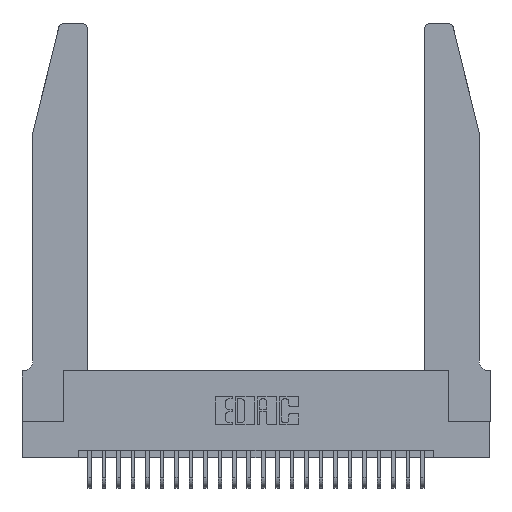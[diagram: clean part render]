
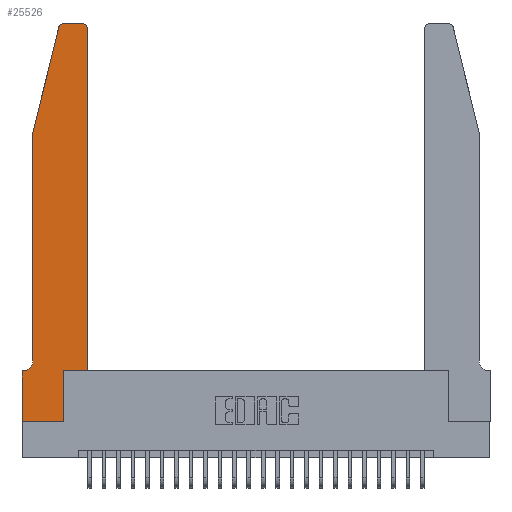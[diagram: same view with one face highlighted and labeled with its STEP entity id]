
A CAD part, top view. The second image highlights one B-rep face of the part: STEP entity #25526.
In plain terms, the highlighted planar face has unit normal (0, 0, 1).
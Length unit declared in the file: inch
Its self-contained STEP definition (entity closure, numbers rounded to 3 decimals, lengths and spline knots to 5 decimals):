
#238 = CARTESIAN_POINT ( 'NONE',  ( 0.2865, 0.35, 0.37 ) ) ;
#315 = ORIENTED_EDGE ( 'NONE', *, *, #3221, .T. ) ;
#940 = DIRECTION ( 'NONE',  ( -0.239, -0.971, 0. ) ) ;
#980 = LINE ( 'NONE', #2149, #10049 ) ;
#1120 = ORIENTED_EDGE ( 'NONE', *, *, #13554, .T. ) ;
#1288 = ORIENTED_EDGE ( 'NONE', *, *, #10608, .T. ) ;
#1357 = VECTOR ( 'NONE', #27537, 39.37008 ) ;
#1616 = CIRCLE ( 'NONE', #3558, 0.03 ) ;
#2002 = ORIENTED_EDGE ( 'NONE', *, *, #13219, .T. ) ;
#2116 = DIRECTION ( 'NONE',  ( 0., -1., 0. ) ) ;
#2149 = CARTESIAN_POINT ( 'NONE',  ( 0.4505, 0.35, 0.37 ) ) ;
#2176 = CARTESIAN_POINT ( 'NONE',  ( 0., 0., 0.37 ) ) ;
#2325 = ORIENTED_EDGE ( 'NONE', *, *, #15446, .T. ) ;
#2406 = EDGE_CURVE ( 'NONE', #17965, #20600, #19378, .T. ) ;
#3221 = EDGE_CURVE ( 'NONE', #5025, #9266, #23312, .T. ) ;
#3550 = VERTEX_POINT ( 'NONE', #16553 ) ;
#3558 = AXIS2_PLACEMENT_3D ( 'NONE', #22043, #26287, #18060 ) ;
#3704 = DIRECTION ( 'NONE',  ( 0., 1., 0. ) ) ;
#4265 = EDGE_CURVE ( 'NONE', #22659, #5025, #15435, .T. ) ;
#4326 = CARTESIAN_POINT ( 'NONE',  ( 0., 0.35, 0.37 ) ) ;
#4814 = LINE ( 'NONE', #26603, #12857 ) ;
#4916 = CARTESIAN_POINT ( 'NONE',  ( 0.4505, 2.72, 0.37 ) ) ;
#4951 = VECTOR ( 'NONE', #3704, 39.37008 ) ;
#5025 = VERTEX_POINT ( 'NONE', #4326 ) ;
#5182 = CARTESIAN_POINT ( 'NONE',  ( 0.0755, 2., 0.37 ) ) ;
#5240 = ORIENTED_EDGE ( 'NONE', *, *, #4265, .T. ) ;
#5340 = LINE ( 'NONE', #8900, #21389 ) ;
#6276 = DIRECTION ( 'NONE',  ( 0., 0., -1. ) ) ;
#8900 = CARTESIAN_POINT ( 'NONE',  ( 0.4505, 0.35, 0.37 ) ) ;
#8917 = CIRCLE ( 'NONE', #25236, 0.03 ) ;
#9266 = VERTEX_POINT ( 'NONE', #20901 ) ;
#9493 = CARTESIAN_POINT ( 'NONE',  ( 0.0055, 0.35, 0.37 ) ) ;
#9686 = ORIENTED_EDGE ( 'NONE', *, *, #2406, .T. ) ;
#10049 = VECTOR ( 'NONE', #25887, 39.37008 ) ;
#10050 = CARTESIAN_POINT ( 'NONE',  ( 0.4505, 0.35, 0.37 ) ) ;
#10266 = CARTESIAN_POINT ( 'NONE',  ( 0., 0., 0.37 ) ) ;
#10285 = EDGE_CURVE ( 'NONE', #14679, #10749, #21225, .T. ) ;
#10608 = EDGE_CURVE ( 'NONE', #19831, #22659, #23866, .T. ) ;
#10749 = VERTEX_POINT ( 'NONE', #20381 ) ;
#10886 = EDGE_CURVE ( 'NONE', #3550, #19831, #4814, .T. ) ;
#11012 = VERTEX_POINT ( 'NONE', #11297 ) ;
#11286 = EDGE_LOOP ( 'NONE', ( #25298, #2325, #15793, #12590, #1288, #5240, #315, #16983, #9686, #2002, #1120, #18285 ) ) ;
#11297 = CARTESIAN_POINT ( 'NONE',  ( 0.25487, 2.72718, 0.37 ) ) ;
#11981 = VECTOR ( 'NONE', #2116, 39.37008 ) ;
#12291 = EDGE_CURVE ( 'NONE', #9266, #17965, #23465, .T. ) ;
#12590 = ORIENTED_EDGE ( 'NONE', *, *, #10886, .T. ) ;
#12857 = VECTOR ( 'NONE', #13670, 39.37008 ) ;
#12926 = DIRECTION ( 'NONE',  ( 0., 0., 1. ) ) ;
#13219 = EDGE_CURVE ( 'NONE', #20600, #26727, #980, .T. ) ;
#13227 = AXIS2_PLACEMENT_3D ( 'NONE', #25328, #12926, #23378 ) ;
#13554 = EDGE_CURVE ( 'NONE', #26727, #26286, #5340, .T. ) ;
#13670 = DIRECTION ( 'NONE',  ( 0., -1., 0. ) ) ;
#14099 = DIRECTION ( 'NONE',  ( -1., 0., 0. ) ) ;
#14679 = VERTEX_POINT ( 'NONE', #22268 ) ;
#15435 = LINE ( 'NONE', #26733, #21762 ) ;
#15446 = EDGE_CURVE ( 'NONE', #10749, #11012, #8917, .T. ) ;
#15793 = ORIENTED_EDGE ( 'NONE', *, *, #20184, .T. ) ;
#15958 = CARTESIAN_POINT ( 'NONE',  ( 0.2865, 0., 0.37 ) ) ;
#16525 = CARTESIAN_POINT ( 'NONE',  ( 0.2605, 2.75, 0.37 ) ) ;
#16553 = CARTESIAN_POINT ( 'NONE',  ( 0.0755, 2., 0.37 ) ) ;
#16983 = ORIENTED_EDGE ( 'NONE', *, *, #12291, .T. ) ;
#17284 = CARTESIAN_POINT ( 'NONE',  ( 0.0755, 0.42, 0.37 ) ) ;
#17965 = VERTEX_POINT ( 'NONE', #15958 ) ;
#18060 = DIRECTION ( 'NONE',  ( 1., 0., 0. ) ) ;
#18285 = ORIENTED_EDGE ( 'NONE', *, *, #26398, .T. ) ;
#18532 = DIRECTION ( 'NONE',  ( 1., 0., 0. ) ) ;
#19128 = PLANE ( 'NONE',  #13227 ) ;
#19136 = CARTESIAN_POINT ( 'NONE',  ( 0.0055, 0.42, 0.37 ) ) ;
#19378 = LINE ( 'NONE', #25362, #4951 ) ;
#19831 = VERTEX_POINT ( 'NONE', #17284 ) ;
#20184 = EDGE_CURVE ( 'NONE', #11012, #3550, #27253, .T. ) ;
#20261 = VECTOR ( 'NONE', #27387, 39.37008 ) ;
#20381 = CARTESIAN_POINT ( 'NONE',  ( 0.284, 2.75, 0.37 ) ) ;
#20600 = VERTEX_POINT ( 'NONE', #238 ) ;
#20901 = CARTESIAN_POINT ( 'NONE',  ( 0., 0., 0.37 ) ) ;
#21225 = LINE ( 'NONE', #16525, #20261 ) ;
#21241 = DIRECTION ( 'NONE',  ( -1., 0., 0. ) ) ;
#21389 = VECTOR ( 'NONE', #23849, 39.37008 ) ;
#21561 = VECTOR ( 'NONE', #940, 39.37008 ) ;
#21762 = VECTOR ( 'NONE', #14099, 39.37008 ) ;
#22043 = CARTESIAN_POINT ( 'NONE',  ( 0.4205, 2.72, 0.37 ) ) ;
#22268 = CARTESIAN_POINT ( 'NONE',  ( 0.4205, 2.75, 0.37 ) ) ;
#22659 = VERTEX_POINT ( 'NONE', #9493 ) ;
#22960 = DIRECTION ( 'NONE',  ( 0., 0., 1. ) ) ;
#23312 = LINE ( 'NONE', #10266, #11981 ) ;
#23378 = DIRECTION ( 'NONE',  ( 1., 0., 0. ) ) ;
#23465 = LINE ( 'NONE', #2176, #1357 ) ;
#23849 = DIRECTION ( 'NONE',  ( 0., 1., 0. ) ) ;
#23866 = CIRCLE ( 'NONE', #24469, 0.07 ) ;
#24469 = AXIS2_PLACEMENT_3D ( 'NONE', #19136, #6276, #21241 ) ;
#25236 = AXIS2_PLACEMENT_3D ( 'NONE', #27227, #22960, #18532 ) ;
#25298 = ORIENTED_EDGE ( 'NONE', *, *, #10285, .T. ) ;
#25328 = CARTESIAN_POINT ( 'NONE',  ( 0., 0.35, 0.37 ) ) ;
#25362 = CARTESIAN_POINT ( 'NONE',  ( 0.2865, 0.35, 0.37 ) ) ;
#25526 = ADVANCED_FACE ( 'NONE', ( #26758 ), #19128, .T. ) ;
#25887 = DIRECTION ( 'NONE',  ( 1., 0., 0. ) ) ;
#26286 = VERTEX_POINT ( 'NONE', #4916 ) ;
#26287 = DIRECTION ( 'NONE',  ( 0., 0., 1. ) ) ;
#26398 = EDGE_CURVE ( 'NONE', #26286, #14679, #1616, .T. ) ;
#26603 = CARTESIAN_POINT ( 'NONE',  ( 0.0755, 2., 0.37 ) ) ;
#26727 = VERTEX_POINT ( 'NONE', #10050 ) ;
#26733 = CARTESIAN_POINT ( 'NONE',  ( 0.0755, 0.35, 0.37 ) ) ;
#26758 = FACE_OUTER_BOUND ( 'NONE', #11286, .T. ) ;
#27227 = CARTESIAN_POINT ( 'NONE',  ( 0.284, 2.72, 0.37 ) ) ;
#27253 = LINE ( 'NONE', #5182, #21561 ) ;
#27387 = DIRECTION ( 'NONE',  ( -1., 0., 0. ) ) ;
#27537 = DIRECTION ( 'NONE',  ( 1., 0., 0. ) ) ;
